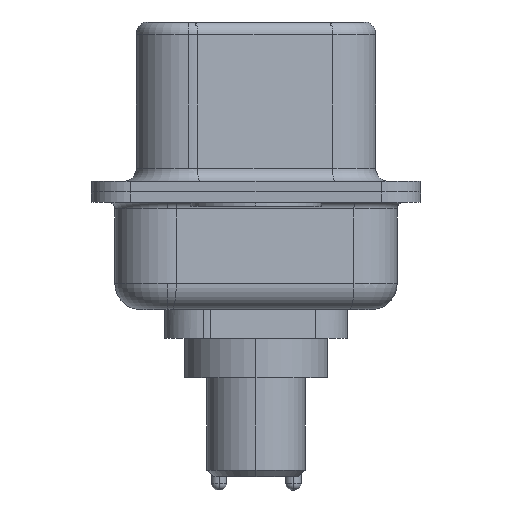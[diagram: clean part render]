
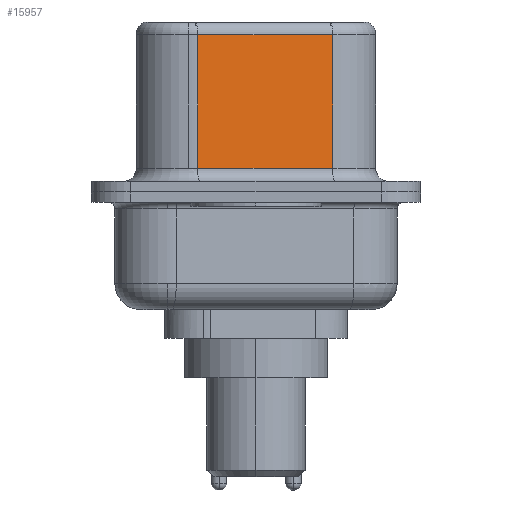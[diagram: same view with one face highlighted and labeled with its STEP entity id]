
A CAD part, left-side view. The second image highlights one B-rep face of the part: STEP entity #15957.
In plain terms, the highlighted planar face has unit normal (-0.985, -0.174, 0).
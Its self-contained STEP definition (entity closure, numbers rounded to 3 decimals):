
#67 = FACE_OUTER_BOUND ( 'NONE', #5940, .T. ) ;
#173 = DIRECTION ( 'NONE',  ( -0.174, 0.985, 0. ) ) ;
#521 = LINE ( 'NONE', #9751, #10744 ) ;
#645 = CARTESIAN_POINT ( 'NONE',  ( 3.67, 2.233, 6.02 ) ) ;
#728 = VECTOR ( 'NONE', #13362, 1000. ) ;
#1277 = DIRECTION ( 'NONE',  ( 0., 0., -1. ) ) ;
#1302 = CARTESIAN_POINT ( 'NONE',  ( 4.58, -2.927, 0.9 ) ) ;
#1449 = CARTESIAN_POINT ( 'NONE',  ( 4.58, -2.927, 6.52 ) ) ;
#2169 = LINE ( 'NONE', #17308, #15554 ) ;
#2667 = CARTESIAN_POINT ( 'NONE',  ( 3.67, 2.233, 6.52 ) ) ;
#2928 = CARTESIAN_POINT ( 'NONE',  ( 4.58, -2.927, 6.02 ) ) ;
#3394 = CARTESIAN_POINT ( 'NONE',  ( 3.67, 2.233, 0.9 ) ) ;
#3860 = DIRECTION ( 'NONE',  ( -0.174, 0.985, 0. ) ) ;
#3980 = VERTEX_POINT ( 'NONE', #14687 ) ;
#4684 = VERTEX_POINT ( 'NONE', #3394 ) ;
#4935 = ORIENTED_EDGE ( 'NONE', *, *, #15417, .T. ) ;
#5169 = ORIENTED_EDGE ( 'NONE', *, *, #7355, .T. ) ;
#5249 = VECTOR ( 'NONE', #3860, 1000. ) ;
#5763 = EDGE_CURVE ( 'NONE', #14978, #4684, #14921, .T. ) ;
#5940 = EDGE_LOOP ( 'NONE', ( #9447, #5169, #11552, #4935 ) ) ;
#7355 = EDGE_CURVE ( 'NONE', #3980, #14978, #15909, .T. ) ;
#8140 = DIRECTION ( 'NONE',  ( 0.985, 0.174, 0. ) ) ;
#9447 = ORIENTED_EDGE ( 'NONE', *, *, #15863, .F. ) ;
#9751 = CARTESIAN_POINT ( 'NONE',  ( 4.58, -2.927, 0.9 ) ) ;
#10744 = VECTOR ( 'NONE', #15112, 1000. ) ;
#11552 = ORIENTED_EDGE ( 'NONE', *, *, #5763, .T. ) ;
#12404 = VERTEX_POINT ( 'NONE', #1302 ) ;
#13362 = DIRECTION ( 'NONE',  ( 0., 0., -1. ) ) ;
#14687 = CARTESIAN_POINT ( 'NONE',  ( 4.58, -2.927, 6.02 ) ) ;
#14921 = LINE ( 'NONE', #2667, #728 ) ;
#14978 = VERTEX_POINT ( 'NONE', #645 ) ;
#15112 = DIRECTION ( 'NONE',  ( 0.174, -0.985, 0. ) ) ;
#15417 = EDGE_CURVE ( 'NONE', #4684, #12404, #521, .T. ) ;
#15554 = VECTOR ( 'NONE', #1277, 1000. ) ;
#15786 = AXIS2_PLACEMENT_3D ( 'NONE', #1449, #8140, #173 ) ;
#15863 = EDGE_CURVE ( 'NONE', #3980, #12404, #2169, .T. ) ;
#15909 = LINE ( 'NONE', #2928, #5249 ) ;
#15957 = ADVANCED_FACE ( 'NONE', ( #67 ), #16175, .F. ) ;
#16175 = PLANE ( 'NONE',  #15786 ) ;
#17308 = CARTESIAN_POINT ( 'NONE',  ( 4.58, -2.927, 6.52 ) ) ;
